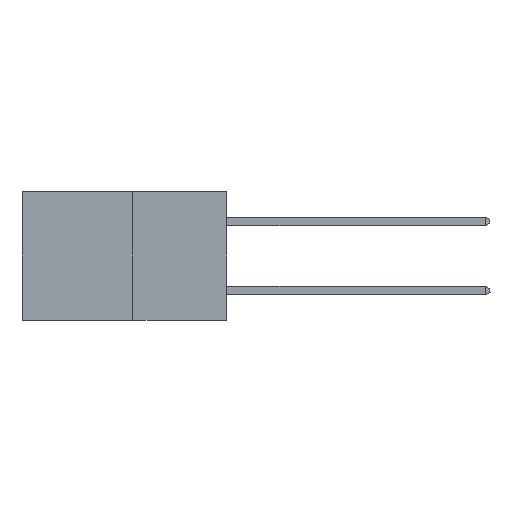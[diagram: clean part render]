
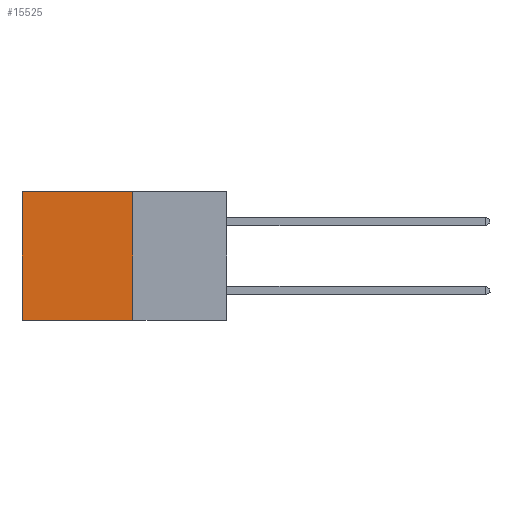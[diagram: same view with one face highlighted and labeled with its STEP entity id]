
A CAD part, left-side view. The second image highlights one B-rep face of the part: STEP entity #15525.
In plain terms, the highlighted planar face has unit normal (-1, 0, 0).
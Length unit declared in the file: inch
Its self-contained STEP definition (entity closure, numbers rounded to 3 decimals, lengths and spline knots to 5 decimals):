
#456 = CARTESIAN_POINT ( 'NONE',  ( 0.277, 0.27, -0.37 ) ) ;
#792 = CARTESIAN_POINT ( 'NONE',  ( 0.277, 0.27, -0.37 ) ) ;
#1170 = ORIENTED_EDGE ( 'NONE', *, *, #14664, .T. ) ;
#1988 = EDGE_CURVE ( 'NONE', #14933, #11516, #8996, .T. ) ;
#2573 = VECTOR ( 'NONE', #10331, 39.37008 ) ;
#3053 = EDGE_LOOP ( 'NONE', ( #1170, #16194, #6115, #9515 ) ) ;
#3271 = VECTOR ( 'NONE', #11366, 39.37008 ) ;
#3519 = CARTESIAN_POINT ( 'NONE',  ( 0.277, 0.27, -0.37 ) ) ;
#3634 = DIRECTION ( 'NONE',  ( 0., 0., -1. ) ) ;
#6115 = ORIENTED_EDGE ( 'NONE', *, *, #10475, .F. ) ;
#6718 = LINE ( 'NONE', #12601, #14509 ) ;
#7545 = VERTEX_POINT ( 'NONE', #10705 ) ;
#8200 = CARTESIAN_POINT ( 'NONE',  ( 0.277, 0.59, 0. ) ) ;
#8996 = LINE ( 'NONE', #12098, #12592 ) ;
#9399 = FACE_OUTER_BOUND ( 'NONE', #3053, .T. ) ;
#9515 = ORIENTED_EDGE ( 'NONE', *, *, #1988, .T. ) ;
#10331 = DIRECTION ( 'NONE',  ( 0., 0., -1. ) ) ;
#10475 = EDGE_CURVE ( 'NONE', #14933, #12977, #12503, .T. ) ;
#10705 = CARTESIAN_POINT ( 'NONE',  ( 0.277, 0.59, -0.37 ) ) ;
#11366 = DIRECTION ( 'NONE',  ( 0., 1., 0. ) ) ;
#11516 = VERTEX_POINT ( 'NONE', #8200 ) ;
#11558 = EDGE_CURVE ( 'NONE', #12977, #7545, #16316, .T. ) ;
#11572 = PLANE ( 'NONE',  #17768 ) ;
#11730 = CARTESIAN_POINT ( 'NONE',  ( 0.277, 0.27, 0. ) ) ;
#11760 = DIRECTION ( 'NONE',  ( 0., 1., 0. ) ) ;
#12098 = CARTESIAN_POINT ( 'NONE',  ( 0.277, 0.27, 0. ) ) ;
#12503 = LINE ( 'NONE', #792, #2573 ) ;
#12592 = VECTOR ( 'NONE', #11760, 39.37008 ) ;
#12601 = CARTESIAN_POINT ( 'NONE',  ( 0.277, 0.59, -0.37 ) ) ;
#12977 = VERTEX_POINT ( 'NONE', #3519 ) ;
#13110 = DIRECTION ( 'NONE',  ( 1., 0., 0. ) ) ;
#14375 = CARTESIAN_POINT ( 'NONE',  ( 0.277, 0.27, -0.37 ) ) ;
#14509 = VECTOR ( 'NONE', #15695, 39.37008 ) ;
#14664 = EDGE_CURVE ( 'NONE', #11516, #7545, #6718, .T. ) ;
#14933 = VERTEX_POINT ( 'NONE', #11730 ) ;
#15525 = ADVANCED_FACE ( 'NONE', ( #9399 ), #11572, .F. ) ;
#15695 = DIRECTION ( 'NONE',  ( 0., 0., -1. ) ) ;
#16194 = ORIENTED_EDGE ( 'NONE', *, *, #11558, .F. ) ;
#16316 = LINE ( 'NONE', #14375, #3271 ) ;
#17768 = AXIS2_PLACEMENT_3D ( 'NONE', #456, #13110, #3634 ) ;
